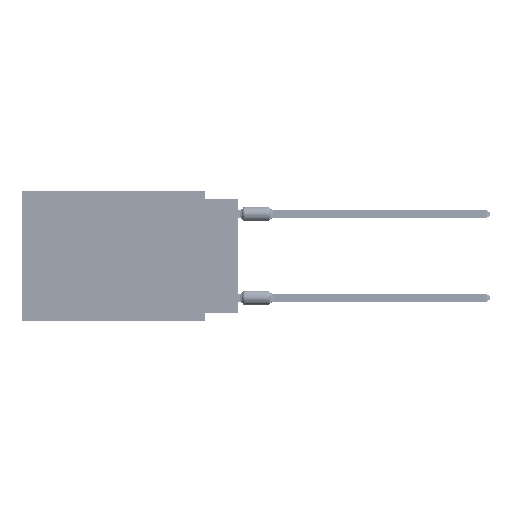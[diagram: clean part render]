
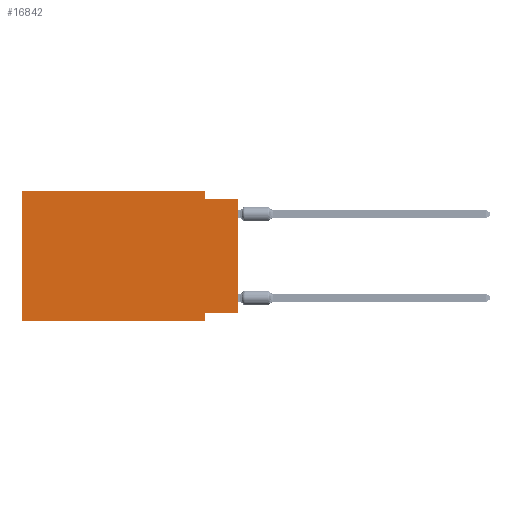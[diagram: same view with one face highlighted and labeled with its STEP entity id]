
A CAD part, left-side view. The second image highlights one B-rep face of the part: STEP entity #16842.
In plain terms, the highlighted planar face has unit normal (-1, 0, 0).
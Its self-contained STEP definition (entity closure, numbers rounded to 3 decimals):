
#740 = EDGE_CURVE ( 'NONE', #82504, #8879, #40369, .T. ) ;
#3061 = VERTEX_POINT ( 'NONE', #70765 ) ;
#3578 = CARTESIAN_POINT ( 'NONE',  ( 0., 2.54, 0. ) ) ;
#5426 = VERTEX_POINT ( 'NONE', #36915 ) ;
#6473 = CARTESIAN_POINT ( 'NONE',  ( 0., 16.383, -9.906 ) ) ;
#7275 = EDGE_CURVE ( 'NONE', #3061, #65292, #20421, .T. ) ;
#7289 = EDGE_CURVE ( 'NONE', #25017, #9143, #72118, .T. ) ;
#8106 = LINE ( 'NONE', #59353, #30667 ) ;
#8879 = VERTEX_POINT ( 'NONE', #26048 ) ;
#9143 = VERTEX_POINT ( 'NONE', #24306 ) ;
#11668 = EDGE_CURVE ( 'NONE', #8879, #9143, #26093, .T. ) ;
#13719 = ORIENTED_EDGE ( 'NONE', *, *, #7275, .F. ) ;
#13764 = CARTESIAN_POINT ( 'NONE',  ( 0., 0., -9.271 ) ) ;
#14642 = CARTESIAN_POINT ( 'NONE',  ( 0., 16.383, 0. ) ) ;
#14880 = DIRECTION ( 'NONE',  ( 0., -1., 0. ) ) ;
#15140 = DIRECTION ( 'NONE',  ( 0., 0., -1. ) ) ;
#15275 = LINE ( 'NONE', #22398, #65666 ) ;
#16201 = AXIS2_PLACEMENT_3D ( 'NONE', #80060, #73355, #35120 ) ;
#16842 = ADVANCED_FACE ( 'NONE', ( #80874 ), #22899, .F. ) ;
#17158 = VECTOR ( 'NONE', #51733, 1000. ) ;
#19834 = ORIENTED_EDGE ( 'NONE', *, *, #11668, .F. ) ;
#20028 = EDGE_CURVE ( 'NONE', #25017, #3061, #53858, .T. ) ;
#20421 = LINE ( 'NONE', #34289, #72268 ) ;
#22398 = CARTESIAN_POINT ( 'NONE',  ( 0., 16.383, -9.906 ) ) ;
#22899 = PLANE ( 'NONE',  #16201 ) ;
#24306 = CARTESIAN_POINT ( 'NONE',  ( 0., 0., -0.635 ) ) ;
#25017 = VERTEX_POINT ( 'NONE', #13764 ) ;
#26048 = CARTESIAN_POINT ( 'NONE',  ( 0., 2.54, -0.635 ) ) ;
#26093 = LINE ( 'NONE', #57220, #17158 ) ;
#27744 = CARTESIAN_POINT ( 'NONE',  ( 0., 2.54, 0. ) ) ;
#28198 = ORIENTED_EDGE ( 'NONE', *, *, #7289, .T. ) ;
#29309 = ORIENTED_EDGE ( 'NONE', *, *, #35383, .F. ) ;
#29882 = ORIENTED_EDGE ( 'NONE', *, *, #20028, .F. ) ;
#30667 = VECTOR ( 'NONE', #45493, 1000. ) ;
#30862 = ORIENTED_EDGE ( 'NONE', *, *, #740, .F. ) ;
#34187 = ORIENTED_EDGE ( 'NONE', *, *, #36012, .T. ) ;
#34289 = CARTESIAN_POINT ( 'NONE',  ( 0., 2.54, -9.906 ) ) ;
#34553 = DIRECTION ( 'NONE',  ( 0., 1., 0. ) ) ;
#35120 = DIRECTION ( 'NONE',  ( 0., 0., -1. ) ) ;
#35383 = EDGE_CURVE ( 'NONE', #5426, #82504, #8106, .T. ) ;
#36012 = EDGE_CURVE ( 'NONE', #54930, #65292, #15275, .T. ) ;
#36915 = CARTESIAN_POINT ( 'NONE',  ( 0., 16.383, 0. ) ) ;
#40369 = LINE ( 'NONE', #27744, #47409 ) ;
#42829 = EDGE_LOOP ( 'NONE', ( #28198, #19834, #30862, #29309, #59913, #34187, #13719, #29882 ) ) ;
#45493 = DIRECTION ( 'NONE',  ( 0., -1., 0. ) ) ;
#47409 = VECTOR ( 'NONE', #15140, 1000. ) ;
#51733 = DIRECTION ( 'NONE',  ( 0., -1., 0. ) ) ;
#53858 = LINE ( 'NONE', #66487, #55603 ) ;
#54254 = EDGE_CURVE ( 'NONE', #54930, #5426, #65920, .T. ) ;
#54930 = VERTEX_POINT ( 'NONE', #6473 ) ;
#55603 = VECTOR ( 'NONE', #34553, 1000. ) ;
#57220 = CARTESIAN_POINT ( 'NONE',  ( 0., 0., -0.635 ) ) ;
#57481 = VECTOR ( 'NONE', #79632, 1000. ) ;
#59353 = CARTESIAN_POINT ( 'NONE',  ( 0., 16.383, 0. ) ) ;
#59498 = DIRECTION ( 'NONE',  ( 0., 0., -1. ) ) ;
#59913 = ORIENTED_EDGE ( 'NONE', *, *, #54254, .F. ) ;
#60728 = CARTESIAN_POINT ( 'NONE',  ( 0., 0., 0. ) ) ;
#60819 = DIRECTION ( 'NONE',  ( 0., 0., 1. ) ) ;
#61402 = VECTOR ( 'NONE', #60819, 1000. ) ;
#65292 = VERTEX_POINT ( 'NONE', #75748 ) ;
#65666 = VECTOR ( 'NONE', #14880, 1000. ) ;
#65920 = LINE ( 'NONE', #14642, #61402 ) ;
#66487 = CARTESIAN_POINT ( 'NONE',  ( 0., 0., -9.271 ) ) ;
#70765 = CARTESIAN_POINT ( 'NONE',  ( 0., 2.54, -9.271 ) ) ;
#72118 = LINE ( 'NONE', #60728, #57481 ) ;
#72268 = VECTOR ( 'NONE', #59498, 1000. ) ;
#73355 = DIRECTION ( 'NONE',  ( 1., 0., 0. ) ) ;
#75748 = CARTESIAN_POINT ( 'NONE',  ( 0., 2.54, -9.906 ) ) ;
#79632 = DIRECTION ( 'NONE',  ( 0., 0., 1. ) ) ;
#80060 = CARTESIAN_POINT ( 'NONE',  ( 0., 16.383, 0. ) ) ;
#80874 = FACE_OUTER_BOUND ( 'NONE', #42829, .T. ) ;
#82504 = VERTEX_POINT ( 'NONE', #3578 ) ;
